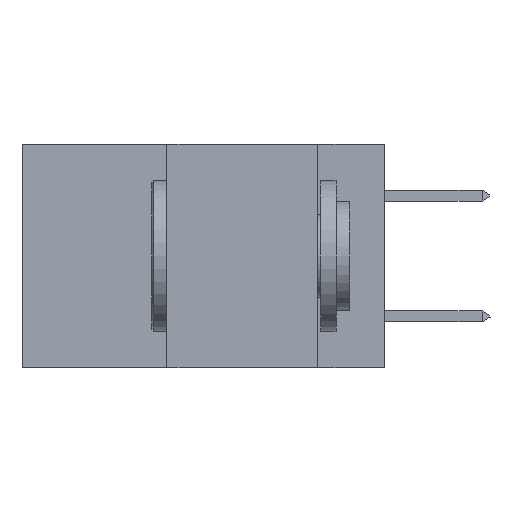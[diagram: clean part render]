
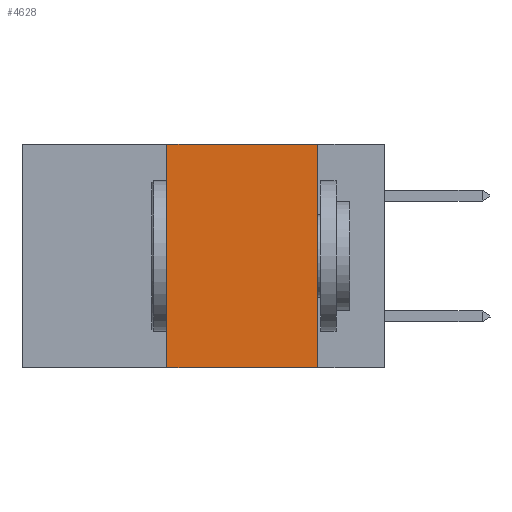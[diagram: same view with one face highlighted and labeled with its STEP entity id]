
A CAD part, left-side view. The second image highlights one B-rep face of the part: STEP entity #4628.
In plain terms, the highlighted planar face has unit normal (-1, 0, 0).
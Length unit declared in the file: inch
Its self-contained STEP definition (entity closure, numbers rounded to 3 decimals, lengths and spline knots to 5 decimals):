
#40 = PLANE ( 'NONE',  #4400 ) ;
#1907 = EDGE_CURVE ( 'NONE', #10456, #8904, #4821, .T. ) ;
#2022 = DIRECTION ( 'NONE',  ( 1., 0., 0. ) ) ;
#2488 = LINE ( 'NONE', #3155, #8059 ) ;
#3033 = DIRECTION ( 'NONE',  ( 0., 0., -1. ) ) ;
#3155 = CARTESIAN_POINT ( 'NONE',  ( 0., 0.6, 0. ) ) ;
#3401 = LINE ( 'NONE', #6147, #5219 ) ;
#4120 = ORIENTED_EDGE ( 'NONE', *, *, #11879, .F. ) ;
#4291 = CARTESIAN_POINT ( 'NONE',  ( 0., 0.11, 0. ) ) ;
#4400 = AXIS2_PLACEMENT_3D ( 'NONE', #10656, #2022, #3033 ) ;
#4628 = ADVANCED_FACE ( 'NONE', ( #11884 ), #40, .F. ) ;
#4821 = LINE ( 'NONE', #8569, #10770 ) ;
#5219 = VECTOR ( 'NONE', #8015, 39.37008 ) ;
#6147 = CARTESIAN_POINT ( 'NONE',  ( 0., 0.11, 0. ) ) ;
#6692 = DIRECTION ( 'NONE',  ( 0., -1., 0. ) ) ;
#7927 = VERTEX_POINT ( 'NONE', #8607 ) ;
#8015 = DIRECTION ( 'NONE',  ( 0., 0., -1. ) ) ;
#8059 = VECTOR ( 'NONE', #9862, 39.37008 ) ;
#8569 = CARTESIAN_POINT ( 'NONE',  ( 0., 0.6, -0.37 ) ) ;
#8607 = CARTESIAN_POINT ( 'NONE',  ( 0., 0.36, 0. ) ) ;
#8615 = LINE ( 'NONE', #9182, #9975 ) ;
#8904 = VERTEX_POINT ( 'NONE', #11190 ) ;
#9182 = CARTESIAN_POINT ( 'NONE',  ( 0., 0.36, 0. ) ) ;
#9296 = ORIENTED_EDGE ( 'NONE', *, *, #1907, .T. ) ;
#9862 = DIRECTION ( 'NONE',  ( 0., -1., 0. ) ) ;
#9938 = DIRECTION ( 'NONE',  ( 0., 0., 1. ) ) ;
#9975 = VECTOR ( 'NONE', #9938, 39.37008 ) ;
#10284 = VERTEX_POINT ( 'NONE', #4291 ) ;
#10376 = ORIENTED_EDGE ( 'NONE', *, *, #12325, .F. ) ;
#10456 = VERTEX_POINT ( 'NONE', #10717 ) ;
#10641 = ORIENTED_EDGE ( 'NONE', *, *, #11495, .F. ) ;
#10656 = CARTESIAN_POINT ( 'NONE',  ( 0., 0.6, 0. ) ) ;
#10717 = CARTESIAN_POINT ( 'NONE',  ( 0., 0.36, -0.37 ) ) ;
#10770 = VECTOR ( 'NONE', #6692, 39.37008 ) ;
#11046 = EDGE_LOOP ( 'NONE', ( #4120, #10641, #10376, #9296 ) ) ;
#11190 = CARTESIAN_POINT ( 'NONE',  ( 0., 0.11, -0.37 ) ) ;
#11495 = EDGE_CURVE ( 'NONE', #7927, #10284, #2488, .T. ) ;
#11879 = EDGE_CURVE ( 'NONE', #10284, #8904, #3401, .T. ) ;
#11884 = FACE_OUTER_BOUND ( 'NONE', #11046, .T. ) ;
#12325 = EDGE_CURVE ( 'NONE', #10456, #7927, #8615, .T. ) ;
